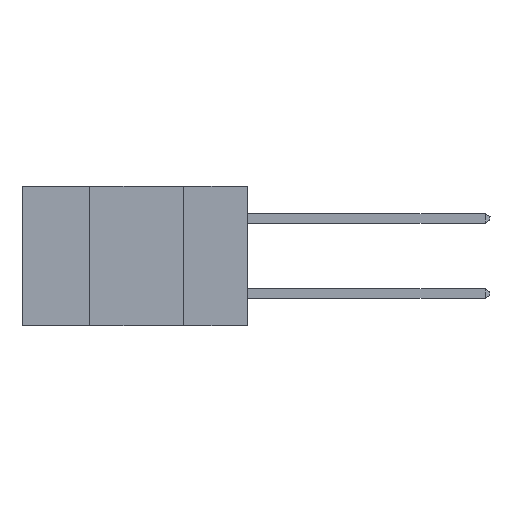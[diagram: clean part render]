
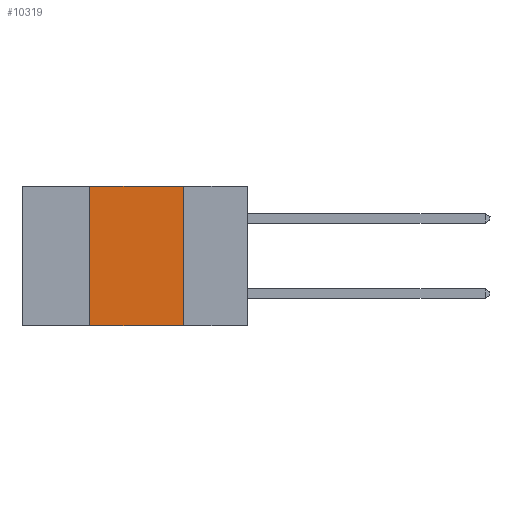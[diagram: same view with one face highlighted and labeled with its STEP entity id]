
A CAD part, left-side view. The second image highlights one B-rep face of the part: STEP entity #10319.
In plain terms, the highlighted planar face has unit normal (-1, 0, 0).
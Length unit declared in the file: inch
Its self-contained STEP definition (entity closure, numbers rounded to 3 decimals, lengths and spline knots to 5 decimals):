
#182 = CARTESIAN_POINT ( 'NONE',  ( 0., 0.6, 0. ) ) ;
#1548 = LINE ( 'NONE', #10122, #12850 ) ;
#2965 = ORIENTED_EDGE ( 'NONE', *, *, #8021, .F. ) ;
#2994 = VERTEX_POINT ( 'NONE', #5353 ) ;
#4550 = FACE_OUTER_BOUND ( 'NONE', #12739, .T. ) ;
#4972 = ORIENTED_EDGE ( 'NONE', *, *, #5997, .F. ) ;
#5353 = CARTESIAN_POINT ( 'NONE',  ( 0., 0.17, -0.37 ) ) ;
#5715 = VECTOR ( 'NONE', #15967, 39.37008 ) ;
#5962 = VECTOR ( 'NONE', #21916, 39.37008 ) ;
#5997 = EDGE_CURVE ( 'NONE', #12025, #2994, #1548, .T. ) ;
#7322 = CARTESIAN_POINT ( 'NONE',  ( 0., 0.17, 0. ) ) ;
#8021 = EDGE_CURVE ( 'NONE', #12515, #12025, #12358, .T. ) ;
#10122 = CARTESIAN_POINT ( 'NONE',  ( 0., 0.17, 0. ) ) ;
#10229 = CARTESIAN_POINT ( 'NONE',  ( 0., 0.6, -0.37 ) ) ;
#10319 = ADVANCED_FACE ( 'NONE', ( #4550 ), #23416, .F. ) ;
#11402 = ORIENTED_EDGE ( 'NONE', *, *, #27333, .F. ) ;
#11751 = DIRECTION ( 'NONE',  ( 0., 0., -1. ) ) ;
#12025 = VERTEX_POINT ( 'NONE', #7322 ) ;
#12261 = ORIENTED_EDGE ( 'NONE', *, *, #25865, .T. ) ;
#12358 = LINE ( 'NONE', #182, #5715 ) ;
#12374 = DIRECTION ( 'NONE',  ( 0., 0., -1. ) ) ;
#12515 = VERTEX_POINT ( 'NONE', #22084 ) ;
#12739 = EDGE_LOOP ( 'NONE', ( #4972, #2965, #11402, #12261 ) ) ;
#12850 = VECTOR ( 'NONE', #11751, 39.37008 ) ;
#12883 = CARTESIAN_POINT ( 'NONE',  ( 0., 0.42, 0. ) ) ;
#15967 = DIRECTION ( 'NONE',  ( 0., -1., 0. ) ) ;
#16768 = CARTESIAN_POINT ( 'NONE',  ( 0., 0.6, 0. ) ) ;
#17583 = VERTEX_POINT ( 'NONE', #28091 ) ;
#17586 = LINE ( 'NONE', #10229, #22744 ) ;
#19940 = AXIS2_PLACEMENT_3D ( 'NONE', #16768, #25607, #12374 ) ;
#21916 = DIRECTION ( 'NONE',  ( 0., 0., 1. ) ) ;
#22084 = CARTESIAN_POINT ( 'NONE',  ( 0., 0.42, 0. ) ) ;
#22744 = VECTOR ( 'NONE', #27889, 39.37008 ) ;
#23416 = PLANE ( 'NONE',  #19940 ) ;
#24372 = LINE ( 'NONE', #12883, #5962 ) ;
#25607 = DIRECTION ( 'NONE',  ( 1., 0., 0. ) ) ;
#25865 = EDGE_CURVE ( 'NONE', #17583, #2994, #17586, .T. ) ;
#27333 = EDGE_CURVE ( 'NONE', #17583, #12515, #24372, .T. ) ;
#27889 = DIRECTION ( 'NONE',  ( 0., -1., 0. ) ) ;
#28091 = CARTESIAN_POINT ( 'NONE',  ( 0., 0.42, -0.37 ) ) ;
